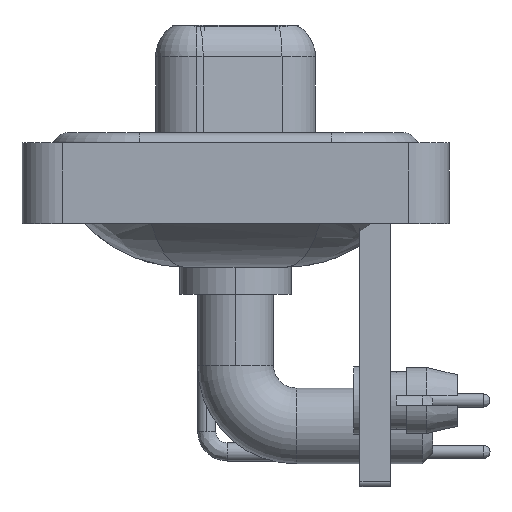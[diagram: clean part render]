
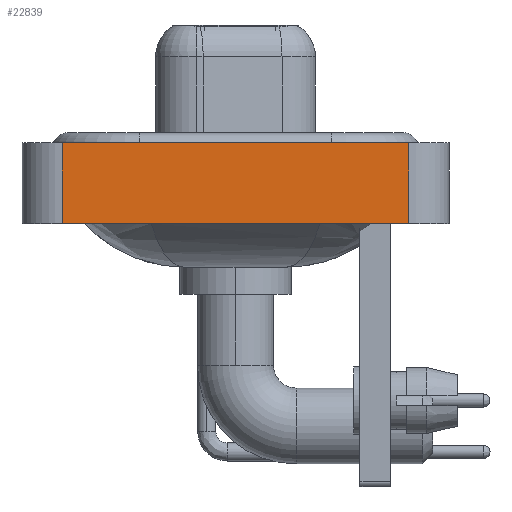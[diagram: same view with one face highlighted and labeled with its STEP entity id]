
A CAD part, left-side view. The second image highlights one B-rep face of the part: STEP entity #22839.
In plain terms, the highlighted planar face has unit normal (-1, 0, 0).
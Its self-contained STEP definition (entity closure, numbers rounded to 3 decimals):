
#430 = CARTESIAN_POINT ( 'NONE',  ( -7.35, -8.55, 0.4 ) ) ;
#447 = LINE ( 'NONE', #4564, #21999 ) ;
#923 = EDGE_CURVE ( 'NONE', #12642, #19972, #9879, .T. ) ;
#966 = VECTOR ( 'NONE', #17745, 1000. ) ;
#1088 = PLANE ( 'NONE',  #22469 ) ;
#2146 = LINE ( 'NONE', #11584, #966 ) ;
#2557 = CARTESIAN_POINT ( 'NONE',  ( -7.35, -8.55, -3.6 ) ) ;
#2639 = ORIENTED_EDGE ( 'NONE', *, *, #12536, .F. ) ;
#2691 = DIRECTION ( 'NONE',  ( 0., -1., 0. ) ) ;
#3263 = DIRECTION ( 'NONE',  ( 0., 0., 1. ) ) ;
#3639 = DIRECTION ( 'NONE',  ( -1., 0., 0. ) ) ;
#4564 = CARTESIAN_POINT ( 'NONE',  ( -7.35, 8.55, -3.6 ) ) ;
#4860 = ORIENTED_EDGE ( 'NONE', *, *, #10340, .T. ) ;
#5297 = EDGE_LOOP ( 'NONE', ( #11035, #19067, #2639, #4860 ) ) ;
#8254 = DIRECTION ( 'NONE',  ( 0., 0., 1. ) ) ;
#9590 = VECTOR ( 'NONE', #23774, 1000. ) ;
#9697 = VERTEX_POINT ( 'NONE', #19735 ) ;
#9879 = LINE ( 'NONE', #430, #9590 ) ;
#10340 = EDGE_CURVE ( 'NONE', #24480, #9697, #11864, .T. ) ;
#11035 = ORIENTED_EDGE ( 'NONE', *, *, #17323, .T. ) ;
#11584 = CARTESIAN_POINT ( 'NONE',  ( -7.35, -8.55, -3.6 ) ) ;
#11864 = LINE ( 'NONE', #2557, #24566 ) ;
#12536 = EDGE_CURVE ( 'NONE', #24480, #12642, #447, .T. ) ;
#12642 = VERTEX_POINT ( 'NONE', #21288 ) ;
#14746 = CARTESIAN_POINT ( 'NONE',  ( -7.35, -8.55, -3.6 ) ) ;
#17323 = EDGE_CURVE ( 'NONE', #9697, #19972, #2146, .T. ) ;
#17745 = DIRECTION ( 'NONE',  ( 0., 0., 1. ) ) ;
#18577 = FACE_OUTER_BOUND ( 'NONE', #5297, .T. ) ;
#19067 = ORIENTED_EDGE ( 'NONE', *, *, #923, .F. ) ;
#19574 = CARTESIAN_POINT ( 'NONE',  ( -7.35, -8.55, 0.4 ) ) ;
#19735 = CARTESIAN_POINT ( 'NONE',  ( -7.35, -8.55, -3.6 ) ) ;
#19972 = VERTEX_POINT ( 'NONE', #19574 ) ;
#21288 = CARTESIAN_POINT ( 'NONE',  ( -7.35, 8.55, 0.4 ) ) ;
#21999 = VECTOR ( 'NONE', #8254, 1000. ) ;
#22469 = AXIS2_PLACEMENT_3D ( 'NONE', #14746, #3639, #3263 ) ;
#22839 = ADVANCED_FACE ( 'NONE', ( #18577 ), #1088, .T. ) ;
#23774 = DIRECTION ( 'NONE',  ( 0., -1., 0. ) ) ;
#24480 = VERTEX_POINT ( 'NONE', #25229 ) ;
#24566 = VECTOR ( 'NONE', #2691, 1000. ) ;
#25229 = CARTESIAN_POINT ( 'NONE',  ( -7.35, 8.55, -3.6 ) ) ;
